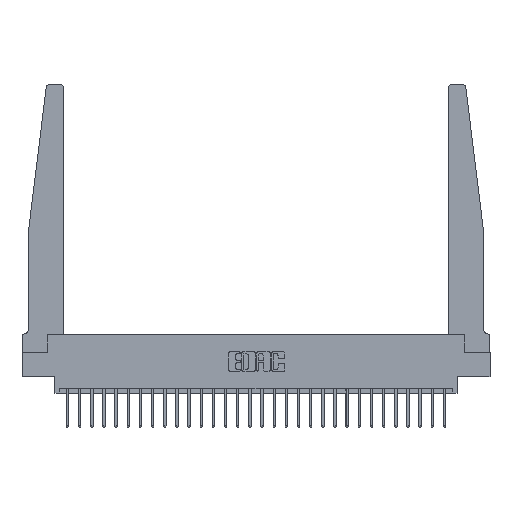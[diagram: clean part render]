
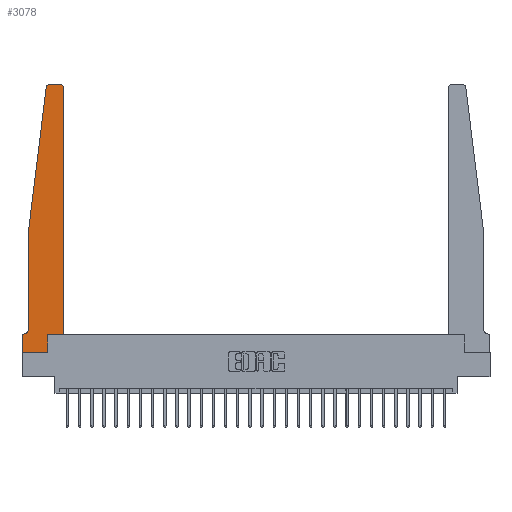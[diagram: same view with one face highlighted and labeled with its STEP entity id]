
A CAD part, top view. The second image highlights one B-rep face of the part: STEP entity #3078.
In plain terms, the highlighted planar face has unit normal (0, 0, 1).
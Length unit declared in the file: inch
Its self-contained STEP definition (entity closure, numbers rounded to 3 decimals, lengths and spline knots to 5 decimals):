
#89 = CARTESIAN_POINT ( 'NONE',  ( 0.015, 0.1875, 0.37 ) ) ;
#318 = ORIENTED_EDGE ( 'NONE', *, *, #605, .T. ) ;
#516 = EDGE_CURVE ( 'NONE', #6795, #6791, #20558, .T. ) ;
#605 = EDGE_CURVE ( 'NONE', #19849, #10499, #21517, .T. ) ;
#942 = CARTESIAN_POINT ( 'NONE',  ( 0.065, 0.1875, 0.37 ) ) ;
#1610 = DIRECTION ( 'NONE',  ( 0., 0., -1. ) ) ;
#1738 = DIRECTION ( 'NONE',  ( 1., 0., 0. ) ) ;
#2101 = VECTOR ( 'NONE', #3310, 39.37008 ) ;
#2601 = VERTEX_POINT ( 'NONE', #22723 ) ;
#2739 = VECTOR ( 'NONE', #7488, 39.37008 ) ;
#3078 = ADVANCED_FACE ( 'NONE', ( #24780 ), #11799, .T. ) ;
#3310 = DIRECTION ( 'NONE',  ( 1., 0., 0. ) ) ;
#4285 = DIRECTION ( 'NONE',  ( 0., 1., 0. ) ) ;
#4290 = CARTESIAN_POINT ( 'NONE',  ( 0.425, 0.18, 0.37 ) ) ;
#4401 = EDGE_CURVE ( 'NONE', #10499, #18261, #24270, .T. ) ;
#4803 = VERTEX_POINT ( 'NONE', #15177 ) ;
#5367 = DIRECTION ( 'NONE',  ( 0., 0., 1. ) ) ;
#5517 = CARTESIAN_POINT ( 'NONE',  ( 0.425, 2.72, 0.37 ) ) ;
#5746 = CIRCLE ( 'NONE', #14649, 0.03 ) ;
#5949 = DIRECTION ( 'NONE',  ( 0., 0., 1. ) ) ;
#5975 = EDGE_CURVE ( 'NONE', #18261, #18853, #17022, .T. ) ;
#6105 = AXIS2_PLACEMENT_3D ( 'NONE', #12352, #5949, #1738 ) ;
#6520 = CARTESIAN_POINT ( 'NONE',  ( 0.2605, 0.18, 0.37 ) ) ;
#6766 = CARTESIAN_POINT ( 'NONE',  ( 0.065, 0.2375, 0.37 ) ) ;
#6791 = VERTEX_POINT ( 'NONE', #27150 ) ;
#6795 = VERTEX_POINT ( 'NONE', #5517 ) ;
#7488 = DIRECTION ( 'NONE',  ( -1., 0., 0. ) ) ;
#7582 = CARTESIAN_POINT ( 'NONE',  ( 0.425, 0.18, 0.37 ) ) ;
#7621 = VECTOR ( 'NONE', #23594, 39.37008 ) ;
#7731 = DIRECTION ( 'NONE',  ( 1., 0., 0. ) ) ;
#7953 = CARTESIAN_POINT ( 'NONE',  ( 0.065, 1.25, 0.37 ) ) ;
#8406 = ORIENTED_EDGE ( 'NONE', *, *, #27188, .T. ) ;
#9049 = LINE ( 'NONE', #942, #2739 ) ;
#9335 = VECTOR ( 'NONE', #9927, 39.37008 ) ;
#9927 = DIRECTION ( 'NONE',  ( 0., -1., 0. ) ) ;
#10115 = ORIENTED_EDGE ( 'NONE', *, *, #11914, .T. ) ;
#10499 = VERTEX_POINT ( 'NONE', #20262 ) ;
#10688 = ORIENTED_EDGE ( 'NONE', *, *, #4401, .T. ) ;
#11162 = CARTESIAN_POINT ( 'NONE',  ( 0., 0., 0.37 ) ) ;
#11513 = VERTEX_POINT ( 'NONE', #18361 ) ;
#11711 = CARTESIAN_POINT ( 'NONE',  ( 0., 0., 0.37 ) ) ;
#11799 = PLANE ( 'NONE',  #6105 ) ;
#11914 = EDGE_CURVE ( 'NONE', #6791, #11513, #21101, .T. ) ;
#11978 = ORIENTED_EDGE ( 'NONE', *, *, #24458, .T. ) ;
#12286 = EDGE_CURVE ( 'NONE', #11513, #4803, #5746, .T. ) ;
#12352 = CARTESIAN_POINT ( 'NONE',  ( 0., 0.1875, 0.37 ) ) ;
#12496 = VERTEX_POINT ( 'NONE', #19658 ) ;
#12530 = AXIS2_PLACEMENT_3D ( 'NONE', #15967, #5367, #14022 ) ;
#12808 = DIRECTION ( 'NONE',  ( 0., 1., 0. ) ) ;
#13283 = VECTOR ( 'NONE', #16500, 39.37008 ) ;
#13959 = DIRECTION ( 'NONE',  ( 0., 0., 1. ) ) ;
#14022 = DIRECTION ( 'NONE',  ( 1., 0., 0. ) ) ;
#14649 = AXIS2_PLACEMENT_3D ( 'NONE', #24569, #13959, #22469 ) ;
#15177 = CARTESIAN_POINT ( 'NONE',  ( 0.24675, 2.72367, 0.37 ) ) ;
#15471 = EDGE_CURVE ( 'NONE', #19573, #27585, #23619, .T. ) ;
#15617 = VECTOR ( 'NONE', #7731, 39.37008 ) ;
#15694 = ORIENTED_EDGE ( 'NONE', *, *, #21769, .T. ) ;
#15967 = CARTESIAN_POINT ( 'NONE',  ( 0.395, 2.72, 0.37 ) ) ;
#16321 = CARTESIAN_POINT ( 'NONE',  ( 0.065, 1.25, 0.37 ) ) ;
#16414 = DIRECTION ( 'NONE',  ( -1., 0., 0. ) ) ;
#16500 = DIRECTION ( 'NONE',  ( -1., 0., 0. ) ) ;
#17022 = LINE ( 'NONE', #6520, #19152 ) ;
#17751 = CARTESIAN_POINT ( 'NONE',  ( 0.2605, 0.18, 0.37 ) ) ;
#17943 = LINE ( 'NONE', #7582, #15617 ) ;
#18261 = VERTEX_POINT ( 'NONE', #21019 ) ;
#18361 = CARTESIAN_POINT ( 'NONE',  ( 0.27653, 2.75, 0.37 ) ) ;
#18518 = EDGE_CURVE ( 'NONE', #18853, #12496, #17943, .T. ) ;
#18728 = AXIS2_PLACEMENT_3D ( 'NONE', #22983, #1610, #16414 ) ;
#18853 = VERTEX_POINT ( 'NONE', #17751 ) ;
#18860 = DIRECTION ( 'NONE',  ( -0.122, -0.992, 0. ) ) ;
#18902 = CARTESIAN_POINT ( 'NONE',  ( 0., 0.1875, 0.37 ) ) ;
#19152 = VECTOR ( 'NONE', #4285, 39.37008 ) ;
#19573 = VERTEX_POINT ( 'NONE', #6766 ) ;
#19581 = ORIENTED_EDGE ( 'NONE', *, *, #516, .T. ) ;
#19658 = CARTESIAN_POINT ( 'NONE',  ( 0.425, 0.18, 0.37 ) ) ;
#19849 = VERTEX_POINT ( 'NONE', #18902 ) ;
#20262 = CARTESIAN_POINT ( 'NONE',  ( 0., 0., 0.37 ) ) ;
#20421 = VECTOR ( 'NONE', #18860, 39.37008 ) ;
#20558 = CIRCLE ( 'NONE', #12530, 0.03 ) ;
#20676 = LINE ( 'NONE', #7953, #9335 ) ;
#20792 = LINE ( 'NONE', #16321, #20421 ) ;
#21019 = CARTESIAN_POINT ( 'NONE',  ( 0.2605, 0., 0.37 ) ) ;
#21101 = LINE ( 'NONE', #27396, #13283 ) ;
#21269 = ORIENTED_EDGE ( 'NONE', *, *, #18518, .T. ) ;
#21517 = LINE ( 'NONE', #11162, #7621 ) ;
#21769 = EDGE_CURVE ( 'NONE', #27585, #19849, #9049, .T. ) ;
#22469 = DIRECTION ( 'NONE',  ( 1., 0., 0. ) ) ;
#22723 = CARTESIAN_POINT ( 'NONE',  ( 0.065, 1.25, 0.37 ) ) ;
#22879 = EDGE_CURVE ( 'NONE', #4803, #2601, #20792, .T. ) ;
#22983 = CARTESIAN_POINT ( 'NONE',  ( 0.015, 0.2375, 0.37 ) ) ;
#23430 = LINE ( 'NONE', #4290, #27314 ) ;
#23594 = DIRECTION ( 'NONE',  ( 0., -1., 0. ) ) ;
#23619 = CIRCLE ( 'NONE', #18728, 0.05 ) ;
#23859 = ORIENTED_EDGE ( 'NONE', *, *, #12286, .T. ) ;
#23968 = ORIENTED_EDGE ( 'NONE', *, *, #15471, .T. ) ;
#24039 = ORIENTED_EDGE ( 'NONE', *, *, #22879, .T. ) ;
#24270 = LINE ( 'NONE', #11711, #2101 ) ;
#24458 = EDGE_CURVE ( 'NONE', #2601, #19573, #20676, .T. ) ;
#24569 = CARTESIAN_POINT ( 'NONE',  ( 0.27653, 2.72, 0.37 ) ) ;
#24780 = FACE_OUTER_BOUND ( 'NONE', #26517, .T. ) ;
#25882 = ORIENTED_EDGE ( 'NONE', *, *, #5975, .T. ) ;
#26517 = EDGE_LOOP ( 'NONE', ( #10115, #23859, #24039, #11978, #23968, #15694, #318, #10688, #25882, #21269, #8406, #19581 ) ) ;
#27150 = CARTESIAN_POINT ( 'NONE',  ( 0.395, 2.75, 0.37 ) ) ;
#27188 = EDGE_CURVE ( 'NONE', #12496, #6795, #23430, .T. ) ;
#27314 = VECTOR ( 'NONE', #12808, 39.37008 ) ;
#27396 = CARTESIAN_POINT ( 'NONE',  ( 0.25, 2.75, 0.37 ) ) ;
#27585 = VERTEX_POINT ( 'NONE', #89 ) ;
